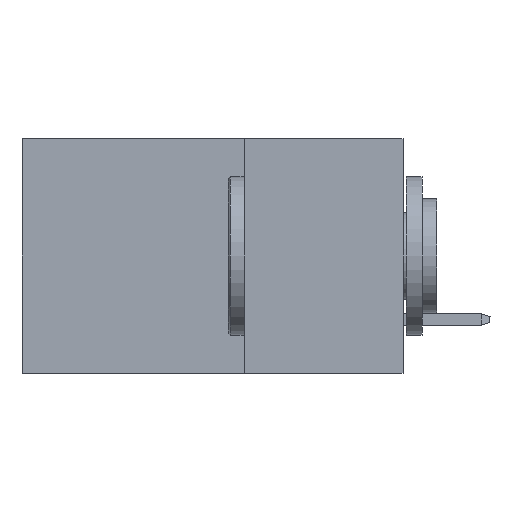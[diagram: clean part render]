
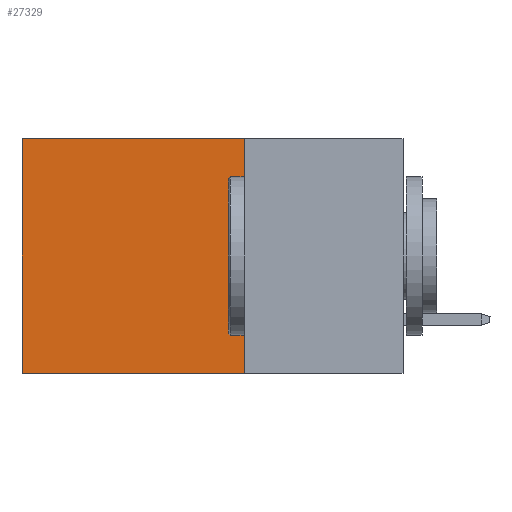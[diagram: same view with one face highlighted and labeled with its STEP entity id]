
A CAD part, left-side view. The second image highlights one B-rep face of the part: STEP entity #27329.
In plain terms, the highlighted planar face has unit normal (-1, 0, 0).
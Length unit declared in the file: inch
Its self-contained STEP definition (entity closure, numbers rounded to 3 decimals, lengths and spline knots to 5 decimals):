
#231 = DIRECTION ( 'NONE',  ( 1., 0., 0. ) ) ;
#557 = CARTESIAN_POINT ( 'NONE',  ( 0.2875, 0.25, 0. ) ) ;
#3484 = ORIENTED_EDGE ( 'NONE', *, *, #13563, .T. ) ;
#4014 = VECTOR ( 'NONE', #30333, 39.37008 ) ;
#7484 = EDGE_CURVE ( 'NONE', #13499, #48410, #18701, .T. ) ;
#7661 = DIRECTION ( 'NONE',  ( 0., 0., -1. ) ) ;
#7902 = FACE_OUTER_BOUND ( 'NONE', #43565, .T. ) ;
#9252 = VERTEX_POINT ( 'NONE', #31967 ) ;
#9539 = ORIENTED_EDGE ( 'NONE', *, *, #34402, .F. ) ;
#10247 = LINE ( 'NONE', #16977, #43544 ) ;
#13086 = VECTOR ( 'NONE', #43821, 39.37008 ) ;
#13499 = VERTEX_POINT ( 'NONE', #29947 ) ;
#13563 = EDGE_CURVE ( 'NONE', #28685, #13499, #26705, .T. ) ;
#13867 = ORIENTED_EDGE ( 'NONE', *, *, #27967, .F. ) ;
#15205 = CARTESIAN_POINT ( 'NONE',  ( 0.2875, 0.6, 0. ) ) ;
#15597 = PLANE ( 'NONE',  #36051 ) ;
#16977 = CARTESIAN_POINT ( 'NONE',  ( 0.2875, 0.25, -0.37 ) ) ;
#17983 = DIRECTION ( 'NONE',  ( 0., 1., 0. ) ) ;
#18701 = LINE ( 'NONE', #15205, #4014 ) ;
#22835 = CARTESIAN_POINT ( 'NONE',  ( 0.2875, 0.25, 0. ) ) ;
#26705 = LINE ( 'NONE', #38100, #36231 ) ;
#27329 = ADVANCED_FACE ( 'NONE', ( #7902 ), #15597, .F. ) ;
#27967 = EDGE_CURVE ( 'NONE', #28685, #9252, #31879, .T. ) ;
#28369 = CARTESIAN_POINT ( 'NONE',  ( 0.2875, 0.6, -0.37 ) ) ;
#28685 = VERTEX_POINT ( 'NONE', #557 ) ;
#29947 = CARTESIAN_POINT ( 'NONE',  ( 0.2875, 0.6, 0. ) ) ;
#30333 = DIRECTION ( 'NONE',  ( 0., 0., -1. ) ) ;
#31597 = ORIENTED_EDGE ( 'NONE', *, *, #7484, .T. ) ;
#31879 = LINE ( 'NONE', #36108, #13086 ) ;
#31967 = CARTESIAN_POINT ( 'NONE',  ( 0.2875, 0.25, -0.37 ) ) ;
#34402 = EDGE_CURVE ( 'NONE', #9252, #48410, #10247, .T. ) ;
#36051 = AXIS2_PLACEMENT_3D ( 'NONE', #22835, #231, #7661 ) ;
#36108 = CARTESIAN_POINT ( 'NONE',  ( 0.2875, 0.25, 0. ) ) ;
#36231 = VECTOR ( 'NONE', #37624, 39.37008 ) ;
#37624 = DIRECTION ( 'NONE',  ( 0., 1., 0. ) ) ;
#38100 = CARTESIAN_POINT ( 'NONE',  ( 0.2875, 0.25, 0. ) ) ;
#43544 = VECTOR ( 'NONE', #17983, 39.37008 ) ;
#43565 = EDGE_LOOP ( 'NONE', ( #31597, #9539, #13867, #3484 ) ) ;
#43821 = DIRECTION ( 'NONE',  ( 0., 0., -1. ) ) ;
#48410 = VERTEX_POINT ( 'NONE', #28369 ) ;
